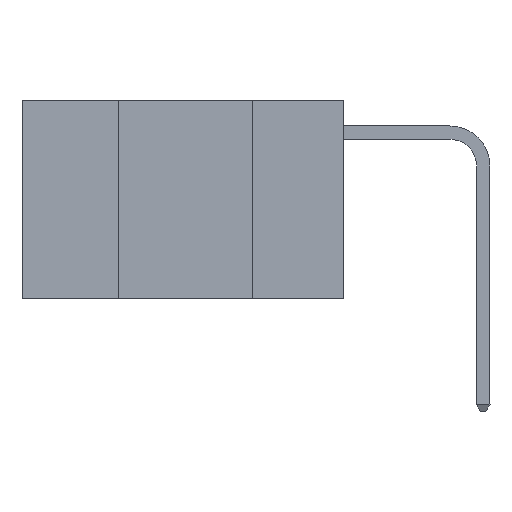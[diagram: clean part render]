
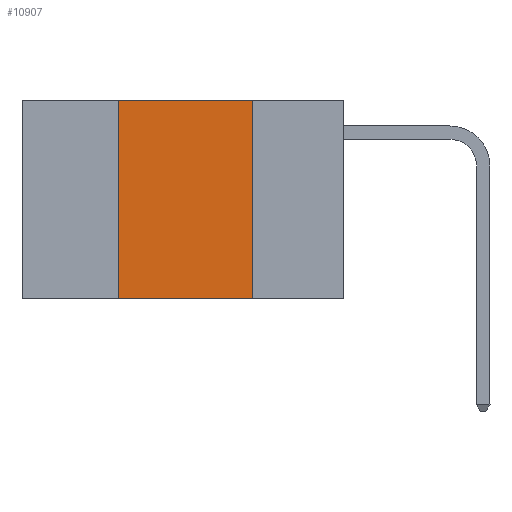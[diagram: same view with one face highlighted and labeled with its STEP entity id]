
A CAD part, left-side view. The second image highlights one B-rep face of the part: STEP entity #10907.
In plain terms, the highlighted planar face has unit normal (-1, 0, 0).
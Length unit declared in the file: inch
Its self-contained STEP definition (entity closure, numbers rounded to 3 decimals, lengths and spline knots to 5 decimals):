
#771 = CARTESIAN_POINT ( 'NONE',  ( 0., 0.6, 0. ) ) ;
#1681 = DIRECTION ( 'NONE',  ( 1., 0., 0. ) ) ;
#1730 = CARTESIAN_POINT ( 'NONE',  ( 0., 0.17, -0.37 ) ) ;
#2111 = CARTESIAN_POINT ( 'NONE',  ( 0., 0.42, 0. ) ) ;
#4194 = FACE_OUTER_BOUND ( 'NONE', #4761, .T. ) ;
#4457 = AXIS2_PLACEMENT_3D ( 'NONE', #4897, #1681, #12799 ) ;
#4761 = EDGE_LOOP ( 'NONE', ( #8959, #9239, #9438, #9561 ) ) ;
#4897 = CARTESIAN_POINT ( 'NONE',  ( 0., 0.6, 0. ) ) ;
#5226 = DIRECTION ( 'NONE',  ( 0., 0., -1. ) ) ;
#5480 = EDGE_CURVE ( 'NONE', #5899, #10480, #13838, .T. ) ;
#5500 = VECTOR ( 'NONE', #13559, 39.37008 ) ;
#5899 = VERTEX_POINT ( 'NONE', #17545 ) ;
#5932 = LINE ( 'NONE', #19193, #14248 ) ;
#6223 = VECTOR ( 'NONE', #5226, 39.37008 ) ;
#6461 = CARTESIAN_POINT ( 'NONE',  ( 0., 0.42, -0.37 ) ) ;
#6591 = EDGE_CURVE ( 'NONE', #10480, #18325, #14527, .T. ) ;
#7702 = VERTEX_POINT ( 'NONE', #6461 ) ;
#8959 = ORIENTED_EDGE ( 'NONE', *, *, #6591, .F. ) ;
#9239 = ORIENTED_EDGE ( 'NONE', *, *, #5480, .F. ) ;
#9438 = ORIENTED_EDGE ( 'NONE', *, *, #19608, .F. ) ;
#9561 = ORIENTED_EDGE ( 'NONE', *, *, #12346, .T. ) ;
#10026 = DIRECTION ( 'NONE',  ( 0., -1., 0. ) ) ;
#10480 = VERTEX_POINT ( 'NONE', #16418 ) ;
#10907 = ADVANCED_FACE ( 'NONE', ( #4194 ), #11202, .F. ) ;
#11202 = PLANE ( 'NONE',  #4457 ) ;
#12346 = EDGE_CURVE ( 'NONE', #7702, #18325, #5932, .T. ) ;
#12612 = LINE ( 'NONE', #2111, #16726 ) ;
#12799 = DIRECTION ( 'NONE',  ( 0., 0., -1. ) ) ;
#13211 = DIRECTION ( 'NONE',  ( 0., 0., 1. ) ) ;
#13559 = DIRECTION ( 'NONE',  ( 0., -1., 0. ) ) ;
#13838 = LINE ( 'NONE', #771, #5500 ) ;
#14248 = VECTOR ( 'NONE', #10026, 39.37008 ) ;
#14527 = LINE ( 'NONE', #17640, #6223 ) ;
#16418 = CARTESIAN_POINT ( 'NONE',  ( 0., 0.17, 0. ) ) ;
#16726 = VECTOR ( 'NONE', #13211, 39.37008 ) ;
#17545 = CARTESIAN_POINT ( 'NONE',  ( 0., 0.42, 0. ) ) ;
#17640 = CARTESIAN_POINT ( 'NONE',  ( 0., 0.17, 0. ) ) ;
#18325 = VERTEX_POINT ( 'NONE', #1730 ) ;
#19193 = CARTESIAN_POINT ( 'NONE',  ( 0., 0.6, -0.37 ) ) ;
#19608 = EDGE_CURVE ( 'NONE', #7702, #5899, #12612, .T. ) ;
